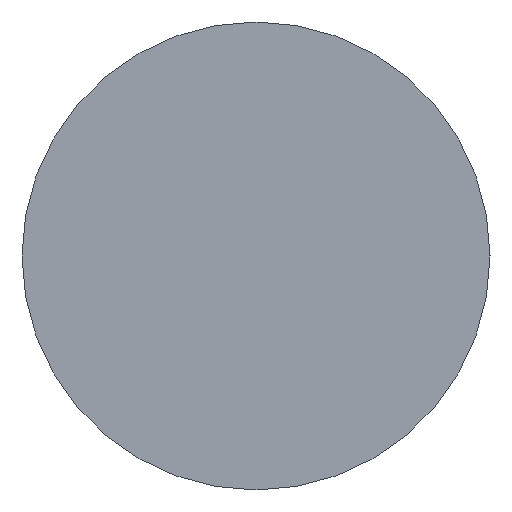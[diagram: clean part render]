
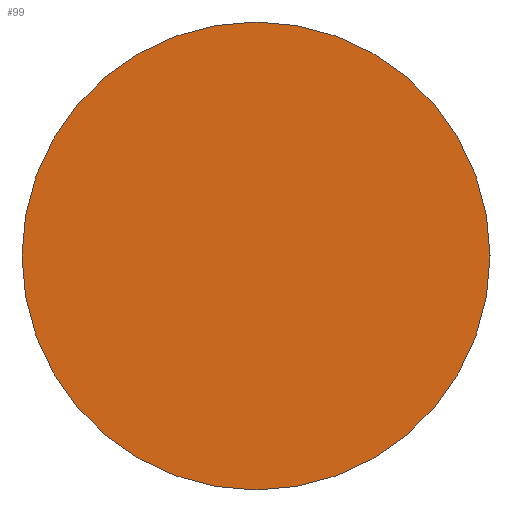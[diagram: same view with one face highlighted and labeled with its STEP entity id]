
A CAD part, left-side view. The second image highlights one B-rep face of the part: STEP entity #99.
In plain terms, the highlighted planar face has unit normal (-1, 0, 0).
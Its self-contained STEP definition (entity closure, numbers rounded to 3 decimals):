
#4 = EDGE_CURVE ( 'NONE', #109, #107, #163, .T. ) ;
#30 = AXIS2_PLACEMENT_3D ( 'NONE', #40, #39, #50 ) ;
#31 = EDGE_CURVE ( 'NONE', #107, #109, #152, .T. ) ;
#35 = AXIS2_PLACEMENT_3D ( 'NONE', #65, #61, #60 ) ;
#36 = AXIS2_PLACEMENT_3D ( 'NONE', #66, #48, #46 ) ;
#39 = DIRECTION ( 'NONE',  ( 1., 0., 0. ) ) ;
#40 = CARTESIAN_POINT ( 'NONE',  ( 0., 0., 0. ) ) ;
#46 = DIRECTION ( 'NONE',  ( 0., 0., -1. ) ) ;
#48 = DIRECTION ( 'NONE',  ( 1., 0., 0. ) ) ;
#50 = DIRECTION ( 'NONE',  ( 0., 0., -1. ) ) ;
#53 = PLANE ( 'NONE',  #36 ) ;
#60 = DIRECTION ( 'NONE',  ( 0., 0., -1. ) ) ;
#61 = DIRECTION ( 'NONE',  ( 1., 0., 0. ) ) ;
#65 = CARTESIAN_POINT ( 'NONE',  ( 0., 0., 0. ) ) ;
#66 = CARTESIAN_POINT ( 'NONE',  ( 0., 0., 0. ) ) ;
#70 = CARTESIAN_POINT ( 'NONE',  ( 0., 0., -2. ) ) ;
#75 = CARTESIAN_POINT ( 'NONE',  ( 0., 0., 2. ) ) ;
#99 = ADVANCED_FACE ( 'NONE', ( #159 ), #53, .F. ) ;
#107 = VERTEX_POINT ( 'NONE', #75 ) ;
#109 = VERTEX_POINT ( 'NONE', #70 ) ;
#120 = ORIENTED_EDGE ( 'NONE', *, *, #4, .F. ) ;
#152 = CIRCLE ( 'NONE', #35, 2. ) ;
#154 = EDGE_LOOP ( 'NONE', ( #160, #120 ) ) ;
#159 = FACE_OUTER_BOUND ( 'NONE', #154, .T. ) ;
#160 = ORIENTED_EDGE ( 'NONE', *, *, #31, .F. ) ;
#163 = CIRCLE ( 'NONE', #30, 2. ) ;
